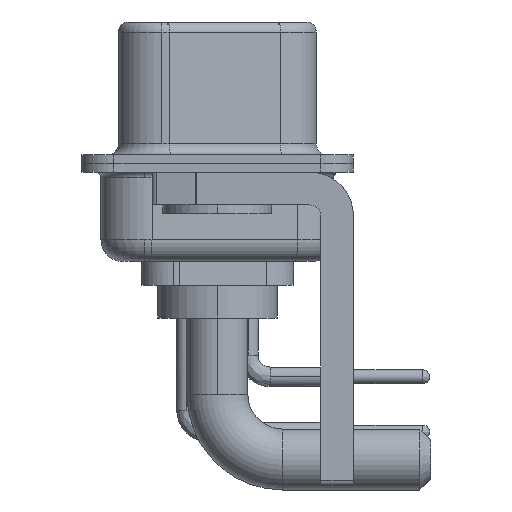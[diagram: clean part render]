
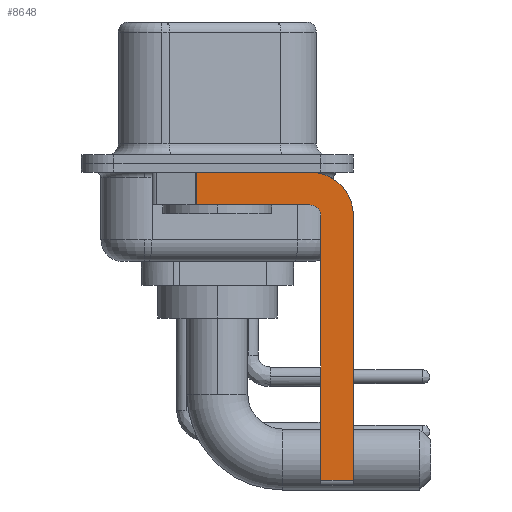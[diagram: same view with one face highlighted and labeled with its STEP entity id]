
A CAD part, left-side view. The second image highlights one B-rep face of the part: STEP entity #8648.
In plain terms, the highlighted planar face has unit normal (-1, 0, 0).
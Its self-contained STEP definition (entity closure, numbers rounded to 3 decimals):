
#246 = VECTOR ( 'NONE', #1067, 1000. ) ;
#287 = EDGE_CURVE ( 'NONE', #14017, #6261, #3275, .T. ) ;
#458 = EDGE_CURVE ( 'NONE', #14017, #23227, #1981, .T. ) ;
#1067 = DIRECTION ( 'NONE',  ( 0., 0., -1. ) ) ;
#1083 = VERTEX_POINT ( 'NONE', #7984 ) ;
#1466 = CARTESIAN_POINT ( 'NONE',  ( -2.9, -4.75, -14.8 ) ) ;
#1492 = ORIENTED_EDGE ( 'NONE', *, *, #22393, .T. ) ;
#1794 = ORIENTED_EDGE ( 'NONE', *, *, #3092, .F. ) ;
#1981 = LINE ( 'NONE', #7765, #3018 ) ;
#2766 = DIRECTION ( 'NONE',  ( 1., 0., 0. ) ) ;
#3018 = VECTOR ( 'NONE', #17072, 1000. ) ;
#3042 = CARTESIAN_POINT ( 'NONE',  ( -2.9, -4.75, -14.55 ) ) ;
#3092 = EDGE_CURVE ( 'NONE', #10637, #14440, #19853, .T. ) ;
#3275 = LINE ( 'NONE', #1466, #14028 ) ;
#3287 = CIRCLE ( 'NONE', #18801, 0.5 ) ;
#3331 = EDGE_CURVE ( 'NONE', #21940, #23227, #20613, .T. ) ;
#3338 = CARTESIAN_POINT ( 'NONE',  ( -2.9, -4.25, -2.4 ) ) ;
#3748 = LINE ( 'NONE', #9518, #19707 ) ;
#4933 = CARTESIAN_POINT ( 'NONE',  ( -2.9, -6.25, -2.4 ) ) ;
#4949 = FACE_OUTER_BOUND ( 'NONE', #7981, .T. ) ;
#5201 = DIRECTION ( 'NONE',  ( -1., 0., 0. ) ) ;
#5843 = CARTESIAN_POINT ( 'NONE',  ( -2.9, 0.978, -1.9 ) ) ;
#6261 = VERTEX_POINT ( 'NONE', #12031 ) ;
#6365 = ORIENTED_EDGE ( 'NONE', *, *, #458, .T. ) ;
#6491 = CARTESIAN_POINT ( 'NONE',  ( -2.9, -4.25, -2.4 ) ) ;
#6629 = DIRECTION ( 'NONE',  ( 0., 0., -1. ) ) ;
#7199 = DIRECTION ( 'NONE',  ( 0., 0., -1. ) ) ;
#7531 = CARTESIAN_POINT ( 'NONE',  ( -2.9, -4.25, -1.9 ) ) ;
#7765 = CARTESIAN_POINT ( 'NONE',  ( -2.9, -4.25, -14.55 ) ) ;
#7981 = EDGE_LOOP ( 'NONE', ( #9630, #1492, #1794, #15721, #10413, #6365, #17380, #12019 ) ) ;
#7984 = CARTESIAN_POINT ( 'NONE',  ( -2.9, 0.978, -0.4 ) ) ;
#8648 = ADVANCED_FACE ( 'NONE', ( #4949 ), #12730, .F. ) ;
#8922 = DIRECTION ( 'NONE',  ( 0., 0., 1. ) ) ;
#9518 = CARTESIAN_POINT ( 'NONE',  ( -2.9, 3., -0.4 ) ) ;
#9630 = ORIENTED_EDGE ( 'NONE', *, *, #17078, .F. ) ;
#9981 = CARTESIAN_POINT ( 'NONE',  ( -2.9, -6.25, -14.55 ) ) ;
#10413 = ORIENTED_EDGE ( 'NONE', *, *, #287, .F. ) ;
#10637 = VERTEX_POINT ( 'NONE', #7531 ) ;
#10879 = DIRECTION ( 'NONE',  ( 1., 0., 0. ) ) ;
#11294 = AXIS2_PLACEMENT_3D ( 'NONE', #6491, #2766, #6629 ) ;
#11550 = DIRECTION ( 'NONE',  ( 0., -1., 0. ) ) ;
#11829 = VECTOR ( 'NONE', #19066, 1000. ) ;
#12019 = ORIENTED_EDGE ( 'NONE', *, *, #22933, .F. ) ;
#12031 = CARTESIAN_POINT ( 'NONE',  ( -2.9, -4.75, -2.4 ) ) ;
#12730 = PLANE ( 'NONE',  #11294 ) ;
#12987 = DIRECTION ( 'NONE',  ( 0., 0., 1. ) ) ;
#14017 = VERTEX_POINT ( 'NONE', #3042 ) ;
#14028 = VECTOR ( 'NONE', #8922, 1000. ) ;
#14240 = CARTESIAN_POINT ( 'NONE',  ( -2.9, 0.978, -1.9 ) ) ;
#14278 = EDGE_CURVE ( 'NONE', #6261, #10637, #3287, .T. ) ;
#14440 = VERTEX_POINT ( 'NONE', #5843 ) ;
#15721 = ORIENTED_EDGE ( 'NONE', *, *, #14278, .F. ) ;
#16297 = CARTESIAN_POINT ( 'NONE',  ( -2.9, -4.25, -1.9 ) ) ;
#16428 = DIRECTION ( 'NONE',  ( 0., 1., 0. ) ) ;
#16749 = AXIS2_PLACEMENT_3D ( 'NONE', #3338, #10879, #7199 ) ;
#17072 = DIRECTION ( 'NONE',  ( 0., -1., 0. ) ) ;
#17078 = EDGE_CURVE ( 'NONE', #1083, #20414, #3748, .T. ) ;
#17380 = ORIENTED_EDGE ( 'NONE', *, *, #3331, .F. ) ;
#18801 = AXIS2_PLACEMENT_3D ( 'NONE', #22679, #5201, #12987 ) ;
#19066 = DIRECTION ( 'NONE',  ( 0., 0., -1. ) ) ;
#19707 = VECTOR ( 'NONE', #11550, 1000. ) ;
#19853 = LINE ( 'NONE', #16297, #22712 ) ;
#20414 = VERTEX_POINT ( 'NONE', #23567 ) ;
#20613 = LINE ( 'NONE', #4933, #246 ) ;
#20796 = CIRCLE ( 'NONE', #16749, 2. ) ;
#21940 = VERTEX_POINT ( 'NONE', #23841 ) ;
#22393 = EDGE_CURVE ( 'NONE', #1083, #14440, #23929, .T. ) ;
#22679 = CARTESIAN_POINT ( 'NONE',  ( -2.9, -4.25, -2.4 ) ) ;
#22712 = VECTOR ( 'NONE', #16428, 1000. ) ;
#22933 = EDGE_CURVE ( 'NONE', #20414, #21940, #20796, .T. ) ;
#23227 = VERTEX_POINT ( 'NONE', #9981 ) ;
#23567 = CARTESIAN_POINT ( 'NONE',  ( -2.9, -4.25, -0.4 ) ) ;
#23841 = CARTESIAN_POINT ( 'NONE',  ( -2.9, -6.25, -2.4 ) ) ;
#23929 = LINE ( 'NONE', #14240, #11829 ) ;
